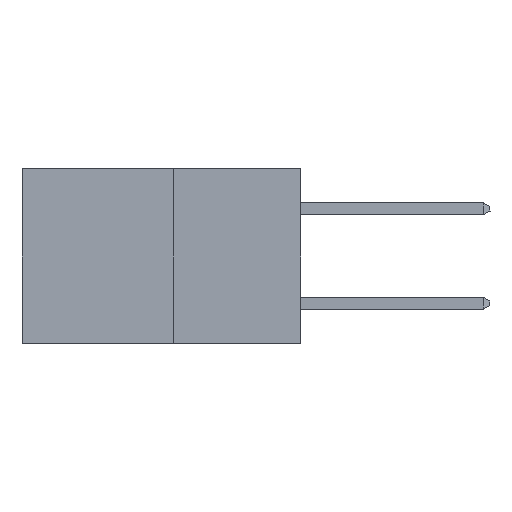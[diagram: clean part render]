
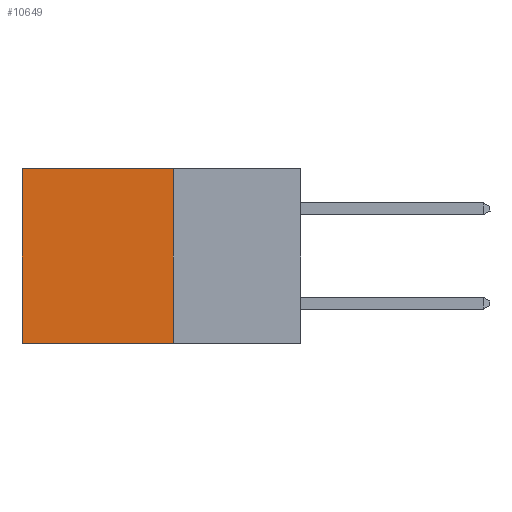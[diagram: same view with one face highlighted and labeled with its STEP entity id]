
A CAD part, left-side view. The second image highlights one B-rep face of the part: STEP entity #10649.
In plain terms, the highlighted planar face has unit normal (-1, 0, 0).
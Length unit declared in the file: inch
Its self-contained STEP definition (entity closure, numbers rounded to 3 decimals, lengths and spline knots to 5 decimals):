
#726 = DIRECTION ( 'NONE',  ( 0., 0., -1. ) ) ;
#1385 = VECTOR ( 'NONE', #1821, 39.37008 ) ;
#1821 = DIRECTION ( 'NONE',  ( 0., 0., -1. ) ) ;
#2044 = CARTESIAN_POINT ( 'NONE',  ( 0.277, 0.27, 0. ) ) ;
#2486 = DIRECTION ( 'NONE',  ( 0., 1., 0. ) ) ;
#4191 = CARTESIAN_POINT ( 'NONE',  ( 0.277, 0.59, 0. ) ) ;
#4675 = EDGE_CURVE ( 'NONE', #11800, #14655, #5361, .T. ) ;
#4804 = EDGE_LOOP ( 'NONE', ( #13109, #6730, #8840, #14126 ) ) ;
#5361 = LINE ( 'NONE', #2044, #18628 ) ;
#5940 = CARTESIAN_POINT ( 'NONE',  ( 0.277, 0.27, -0.37 ) ) ;
#6730 = ORIENTED_EDGE ( 'NONE', *, *, #11354, .F. ) ;
#7054 = CARTESIAN_POINT ( 'NONE',  ( 0.277, 0.59, -0.37 ) ) ;
#7172 = EDGE_CURVE ( 'NONE', #14655, #7887, #19869, .T. ) ;
#7887 = VERTEX_POINT ( 'NONE', #7054 ) ;
#8515 = EDGE_CURVE ( 'NONE', #11800, #18732, #16300, .T. ) ;
#8676 = DIRECTION ( 'NONE',  ( 0., 0., -1. ) ) ;
#8807 = VECTOR ( 'NONE', #2486, 39.37008 ) ;
#8840 = ORIENTED_EDGE ( 'NONE', *, *, #8515, .F. ) ;
#10474 = CARTESIAN_POINT ( 'NONE',  ( 0.277, 0.59, -0.37 ) ) ;
#10649 = ADVANCED_FACE ( 'NONE', ( #19366 ), #21500, .F. ) ;
#10655 = CARTESIAN_POINT ( 'NONE',  ( 0.277, 0.27, -0.37 ) ) ;
#11219 = DIRECTION ( 'NONE',  ( 1., 0., 0. ) ) ;
#11354 = EDGE_CURVE ( 'NONE', #18732, #7887, #13409, .T. ) ;
#11476 = AXIS2_PLACEMENT_3D ( 'NONE', #12865, #11219, #726 ) ;
#11800 = VERTEX_POINT ( 'NONE', #17952 ) ;
#12865 = CARTESIAN_POINT ( 'NONE',  ( 0.277, 0.27, -0.37 ) ) ;
#13109 = ORIENTED_EDGE ( 'NONE', *, *, #7172, .T. ) ;
#13409 = LINE ( 'NONE', #5940, #8807 ) ;
#14126 = ORIENTED_EDGE ( 'NONE', *, *, #4675, .T. ) ;
#14655 = VERTEX_POINT ( 'NONE', #4191 ) ;
#16036 = DIRECTION ( 'NONE',  ( 0., 1., 0. ) ) ;
#16300 = LINE ( 'NONE', #19009, #20334 ) ;
#17952 = CARTESIAN_POINT ( 'NONE',  ( 0.277, 0.27, 0. ) ) ;
#18628 = VECTOR ( 'NONE', #16036, 39.37008 ) ;
#18732 = VERTEX_POINT ( 'NONE', #10655 ) ;
#19009 = CARTESIAN_POINT ( 'NONE',  ( 0.277, 0.27, -0.37 ) ) ;
#19366 = FACE_OUTER_BOUND ( 'NONE', #4804, .T. ) ;
#19869 = LINE ( 'NONE', #10474, #1385 ) ;
#20334 = VECTOR ( 'NONE', #8676, 39.37008 ) ;
#21500 = PLANE ( 'NONE',  #11476 ) ;
